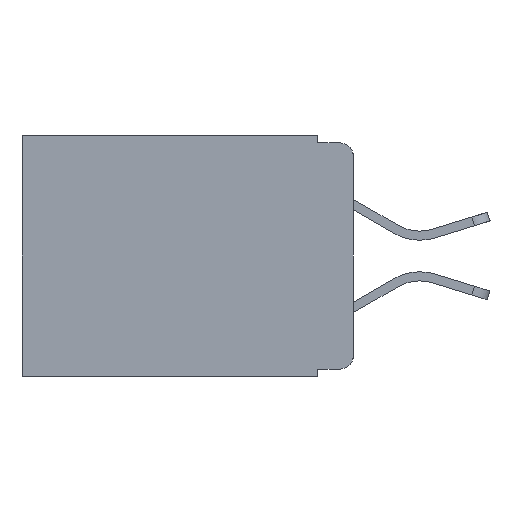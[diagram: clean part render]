
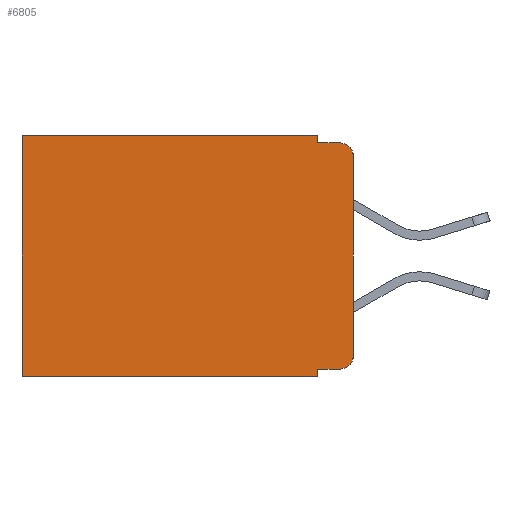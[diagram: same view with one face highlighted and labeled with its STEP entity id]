
A CAD part, left-side view. The second image highlights one B-rep face of the part: STEP entity #6805.
In plain terms, the highlighted planar face has unit normal (-1, 0, 0).
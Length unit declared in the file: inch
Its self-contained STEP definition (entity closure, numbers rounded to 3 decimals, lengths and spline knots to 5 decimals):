
#800 = EDGE_CURVE ( 'NONE', #3595, #14684, #13341, .T. ) ;
#922 = DIRECTION ( 'NONE',  ( 0., 0., -1. ) ) ;
#996 = CARTESIAN_POINT ( 'NONE',  ( 0.298, 0.02, -0.313 ) ) ;
#1232 = LINE ( 'NONE', #3100, #8694 ) ;
#1256 = VERTEX_POINT ( 'NONE', #18356 ) ;
#1459 = DIRECTION ( 'NONE',  ( 0., 0., -1. ) ) ;
#1477 = ORIENTED_EDGE ( 'NONE', *, *, #1958, .F. ) ;
#1741 = CARTESIAN_POINT ( 'NONE',  ( 0.298, 0., -0.03 ) ) ;
#1748 = FACE_OUTER_BOUND ( 'NONE', #16161, .T. ) ;
#1958 = EDGE_CURVE ( 'NONE', #3475, #8475, #2711, .T. ) ;
#2711 = LINE ( 'NONE', #6068, #17192 ) ;
#2892 = AXIS2_PLACEMENT_3D ( 'NONE', #11579, #15926, #5405 ) ;
#2908 = DIRECTION ( 'NONE',  ( 0., 0., -1. ) ) ;
#3100 = CARTESIAN_POINT ( 'NONE',  ( 0.298, 0.473, 0. ) ) ;
#3475 = VERTEX_POINT ( 'NONE', #9486 ) ;
#3507 = ORIENTED_EDGE ( 'NONE', *, *, #7004, .F. ) ;
#3595 = VERTEX_POINT ( 'NONE', #1741 ) ;
#3629 = EDGE_CURVE ( 'NONE', #8475, #6176, #12541, .T. ) ;
#3889 = CARTESIAN_POINT ( 'NONE',  ( 0.298, 0., -0.343 ) ) ;
#4346 = CARTESIAN_POINT ( 'NONE',  ( 0.298, 0.473, 0. ) ) ;
#4420 = PLANE ( 'NONE',  #11527 ) ;
#5197 = DIRECTION ( 'NONE',  ( 0., 0., -1. ) ) ;
#5205 = ORIENTED_EDGE ( 'NONE', *, *, #800, .T. ) ;
#5371 = DIRECTION ( 'NONE',  ( 0., -1., 0. ) ) ;
#5405 = DIRECTION ( 'NONE',  ( 0., 0., -1. ) ) ;
#5531 = CARTESIAN_POINT ( 'NONE',  ( 0.298, 0.473, -0.343 ) ) ;
#5580 = CARTESIAN_POINT ( 'NONE',  ( 0.298, 0.051, -0.01 ) ) ;
#6068 = CARTESIAN_POINT ( 'NONE',  ( 0.298, 0.051, 0. ) ) ;
#6087 = VERTEX_POINT ( 'NONE', #13976 ) ;
#6176 = VERTEX_POINT ( 'NONE', #5531 ) ;
#6805 = ADVANCED_FACE ( 'NONE', ( #1748 ), #4420, .F. ) ;
#6944 = DIRECTION ( 'NONE',  ( -1., 0., 0. ) ) ;
#7004 = EDGE_CURVE ( 'NONE', #3595, #1256, #12743, .T. ) ;
#7799 = DIRECTION ( 'NONE',  ( 1., 0., 0. ) ) ;
#7921 = CARTESIAN_POINT ( 'NONE',  ( 0.298, 0.051, 0. ) ) ;
#8475 = VERTEX_POINT ( 'NONE', #11658 ) ;
#8651 = DIRECTION ( 'NONE',  ( 0., 0., -1. ) ) ;
#8667 = VECTOR ( 'NONE', #5371, 39.37008 ) ;
#8694 = VECTOR ( 'NONE', #2908, 39.37008 ) ;
#8729 = ORIENTED_EDGE ( 'NONE', *, *, #14976, .T. ) ;
#8820 = ORIENTED_EDGE ( 'NONE', *, *, #11445, .F. ) ;
#8917 = EDGE_CURVE ( 'NONE', #13876, #6087, #14494, .T. ) ;
#8925 = CARTESIAN_POINT ( 'NONE',  ( 0.298, 0., 0. ) ) ;
#8942 = EDGE_CURVE ( 'NONE', #13876, #11202, #16278, .T. ) ;
#9486 = CARTESIAN_POINT ( 'NONE',  ( 0.298, 0.051, -0.333 ) ) ;
#9745 = VECTOR ( 'NONE', #14396, 39.37008 ) ;
#9909 = ORIENTED_EDGE ( 'NONE', *, *, #13619, .T. ) ;
#9975 = ORIENTED_EDGE ( 'NONE', *, *, #3629, .F. ) ;
#10148 = CARTESIAN_POINT ( 'NONE',  ( 0.298, 0.051, 0. ) ) ;
#11202 = VERTEX_POINT ( 'NONE', #4346 ) ;
#11218 = CARTESIAN_POINT ( 'NONE',  ( 0.298, 0.051, -0.333 ) ) ;
#11445 = EDGE_CURVE ( 'NONE', #6087, #14684, #17574, .T. ) ;
#11480 = CIRCLE ( 'NONE', #14971, 0.02 ) ;
#11527 = AXIS2_PLACEMENT_3D ( 'NONE', #8925, #7799, #1459 ) ;
#11579 = CARTESIAN_POINT ( 'NONE',  ( 0.298, 0.02, -0.03 ) ) ;
#11658 = CARTESIAN_POINT ( 'NONE',  ( 0.298, 0.051, -0.343 ) ) ;
#12541 = LINE ( 'NONE', #3889, #9745 ) ;
#12743 = LINE ( 'NONE', #18764, #19109 ) ;
#13113 = CARTESIAN_POINT ( 'NONE',  ( 0.298, 0., 0. ) ) ;
#13341 = CIRCLE ( 'NONE', #2892, 0.02 ) ;
#13561 = EDGE_CURVE ( 'NONE', #13828, #1256, #11480, .T. ) ;
#13619 = EDGE_CURVE ( 'NONE', #3475, #13828, #14264, .T. ) ;
#13828 = VERTEX_POINT ( 'NONE', #14049 ) ;
#13876 = VERTEX_POINT ( 'NONE', #7921 ) ;
#13976 = CARTESIAN_POINT ( 'NONE',  ( 0.298, 0.051, -0.01 ) ) ;
#14049 = CARTESIAN_POINT ( 'NONE',  ( 0.298, 0.02, -0.333 ) ) ;
#14264 = LINE ( 'NONE', #11218, #16530 ) ;
#14309 = VECTOR ( 'NONE', #14693, 39.37008 ) ;
#14396 = DIRECTION ( 'NONE',  ( 0., 1., 0. ) ) ;
#14494 = LINE ( 'NONE', #10148, #18755 ) ;
#14684 = VERTEX_POINT ( 'NONE', #18277 ) ;
#14693 = DIRECTION ( 'NONE',  ( 0., 1., 0. ) ) ;
#14971 = AXIS2_PLACEMENT_3D ( 'NONE', #996, #6944, #8651 ) ;
#14976 = EDGE_CURVE ( 'NONE', #11202, #6176, #1232, .T. ) ;
#15061 = ORIENTED_EDGE ( 'NONE', *, *, #8917, .F. ) ;
#15926 = DIRECTION ( 'NONE',  ( -1., 0., 0. ) ) ;
#16080 = ORIENTED_EDGE ( 'NONE', *, *, #8942, .T. ) ;
#16161 = EDGE_LOOP ( 'NONE', ( #3507, #5205, #8820, #15061, #16080, #8729, #9975, #1477, #9909, #18360 ) ) ;
#16278 = LINE ( 'NONE', #13113, #14309 ) ;
#16530 = VECTOR ( 'NONE', #19010, 39.37008 ) ;
#17192 = VECTOR ( 'NONE', #19346, 39.37008 ) ;
#17574 = LINE ( 'NONE', #5580, #8667 ) ;
#18277 = CARTESIAN_POINT ( 'NONE',  ( 0.298, 0.02, -0.01 ) ) ;
#18356 = CARTESIAN_POINT ( 'NONE',  ( 0.298, 0., -0.313 ) ) ;
#18360 = ORIENTED_EDGE ( 'NONE', *, *, #13561, .T. ) ;
#18755 = VECTOR ( 'NONE', #922, 39.37008 ) ;
#18764 = CARTESIAN_POINT ( 'NONE',  ( 0.298, 0., 0. ) ) ;
#19010 = DIRECTION ( 'NONE',  ( 0., -1., 0. ) ) ;
#19109 = VECTOR ( 'NONE', #5197, 39.37008 ) ;
#19346 = DIRECTION ( 'NONE',  ( 0., 0., -1. ) ) ;
